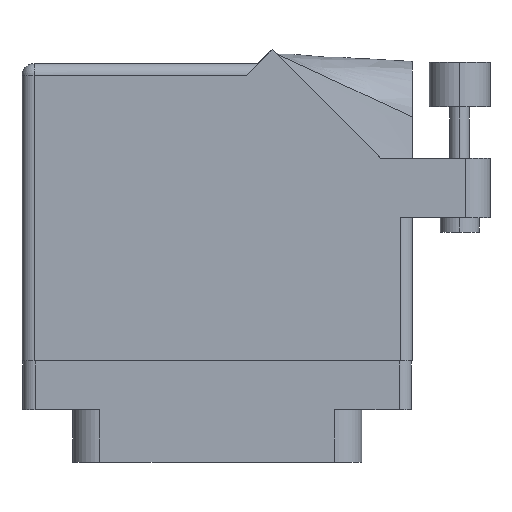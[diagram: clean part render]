
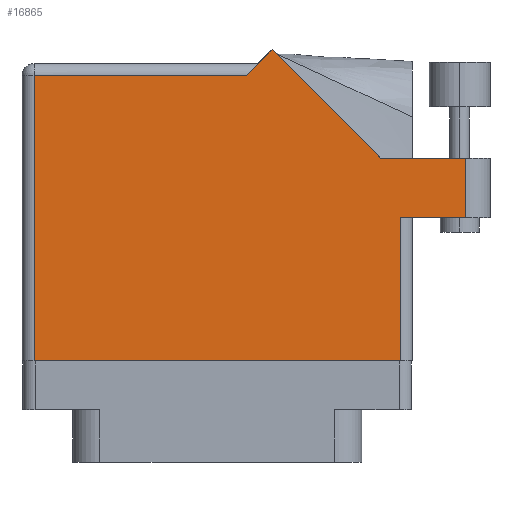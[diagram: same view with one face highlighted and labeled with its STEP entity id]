
A CAD part, front view. The second image highlights one B-rep face of the part: STEP entity #16865.
In plain terms, the highlighted face is planar.
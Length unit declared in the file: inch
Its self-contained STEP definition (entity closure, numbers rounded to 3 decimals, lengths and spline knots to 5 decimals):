
#17 = DIRECTION ( 'NONE',  ( -1., 0., 0. ) ) ;
#161 = VECTOR ( 'NONE', #27261, 39.37008 ) ;
#1463 = CARTESIAN_POINT ( 'NONE',  ( 1.405, 0.944, 0.455 ) ) ;
#2223 = VERTEX_POINT ( 'NONE', #5189 ) ;
#2932 = CARTESIAN_POINT ( 'NONE',  ( 0.83942, 0.944, 0.455 ) ) ;
#3528 = CARTESIAN_POINT ( 'NONE',  ( 1.28, 0.637, 0.455 ) ) ;
#3667 = VECTOR ( 'NONE', #25063, 39.37008 ) ;
#4051 = LINE ( 'NONE', #40041, #161 ) ;
#4214 = FACE_OUTER_BOUND ( 'NONE', #16245, .T. ) ;
#4226 = CARTESIAN_POINT ( 'NONE',  ( 0.943, 0.637, 0.455 ) ) ;
#4454 = DIRECTION ( 'NONE',  ( -1., 0., 0. ) ) ;
#4466 = CARTESIAN_POINT ( 'NONE',  ( 0.15, 1.368, 0.455 ) ) ;
#4490 = EDGE_CURVE ( 'NONE', #36131, #19155, #18329, .T. ) ;
#5189 = CARTESIAN_POINT ( 'NONE',  ( -0.943, 1.368, 0.455 ) ) ;
#6384 = VERTEX_POINT ( 'NONE', #32103 ) ;
#6926 = VERTEX_POINT ( 'NONE', #20071 ) ;
#7021 = VECTOR ( 'NONE', #33291, 39.37008 ) ;
#7250 = ORIENTED_EDGE ( 'NONE', *, *, #4490, .T. ) ;
#8870 = EDGE_CURVE ( 'NONE', #21446, #2223, #4051, .T. ) ;
#8940 = EDGE_CURVE ( 'NONE', #39528, #6384, #28328, .T. ) ;
#10396 = ORIENTED_EDGE ( 'NONE', *, *, #32902, .T. ) ;
#11553 = EDGE_CURVE ( 'NONE', #19155, #21446, #32974, .T. ) ;
#13306 = DIRECTION ( 'NONE',  ( -0.707, -0.707, 0. ) ) ;
#13759 = ORIENTED_EDGE ( 'NONE', *, *, #15859, .T. ) ;
#14920 = VERTEX_POINT ( 'NONE', #26353 ) ;
#15398 = ORIENTED_EDGE ( 'NONE', *, *, #8870, .T. ) ;
#15599 = PLANE ( 'NONE',  #40163 ) ;
#15859 = EDGE_CURVE ( 'NONE', #14920, #34988, #20311, .T. ) ;
#16245 = EDGE_LOOP ( 'NONE', ( #18199, #21356, #18265, #7250, #24539, #15398, #27740, #10396, #13759 ) ) ;
#16865 = ADVANCED_FACE ( 'NONE', ( #4214 ), #15599, .F. ) ;
#16963 = LINE ( 'NONE', #31550, #29628 ) ;
#17164 = DIRECTION ( 'NONE',  ( -0.707, 0.707, 0. ) ) ;
#17356 = EDGE_CURVE ( 'NONE', #34988, #39528, #27983, .T. ) ;
#18199 = ORIENTED_EDGE ( 'NONE', *, *, #17356, .T. ) ;
#18265 = ORIENTED_EDGE ( 'NONE', *, *, #26568, .T. ) ;
#18314 = LINE ( 'NONE', #1463, #38742 ) ;
#18329 = LINE ( 'NONE', #26810, #19810 ) ;
#19155 = VERTEX_POINT ( 'NONE', #21959 ) ;
#19273 = CARTESIAN_POINT ( 'NONE',  ( 0.943, 0.637, 0.455 ) ) ;
#19670 = DIRECTION ( 'NONE',  ( 0., 1., 0. ) ) ;
#19810 = VECTOR ( 'NONE', #17164, 39.37008 ) ;
#20071 = CARTESIAN_POINT ( 'NONE',  ( -0.943, -0.1, 0.455 ) ) ;
#20311 = LINE ( 'NONE', #19273, #31012 ) ;
#20610 = LINE ( 'NONE', #21045, #7021 ) ;
#21045 = CARTESIAN_POINT ( 'NONE',  ( -0.943, -0.1, 0.455 ) ) ;
#21356 = ORIENTED_EDGE ( 'NONE', *, *, #8940, .T. ) ;
#21446 = VERTEX_POINT ( 'NONE', #4466 ) ;
#21959 = CARTESIAN_POINT ( 'NONE',  ( 0.28271, 1.50071, 0.455 ) ) ;
#24539 = ORIENTED_EDGE ( 'NONE', *, *, #11553, .T. ) ;
#25014 = DIRECTION ( 'NONE',  ( 1., 0., 0. ) ) ;
#25063 = DIRECTION ( 'NONE',  ( 1., 0., 0. ) ) ;
#25674 = CARTESIAN_POINT ( 'NONE',  ( 0.212, 1.43, 0.455 ) ) ;
#26353 = CARTESIAN_POINT ( 'NONE',  ( 0.943, -0.1, 0.455 ) ) ;
#26568 = EDGE_CURVE ( 'NONE', #6384, #36131, #18314, .T. ) ;
#26810 = CARTESIAN_POINT ( 'NONE',  ( 0.83942, 0.944, 0.455 ) ) ;
#27261 = DIRECTION ( 'NONE',  ( -1., 0., 0. ) ) ;
#27740 = ORIENTED_EDGE ( 'NONE', *, *, #38437, .T. ) ;
#27983 = LINE ( 'NONE', #28462, #3667 ) ;
#28328 = LINE ( 'NONE', #37324, #29767 ) ;
#28462 = CARTESIAN_POINT ( 'NONE',  ( 1.005, 0.637, 0.455 ) ) ;
#29628 = VECTOR ( 'NONE', #25014, 39.37008 ) ;
#29767 = VECTOR ( 'NONE', #34321, 39.37008 ) ;
#31012 = VECTOR ( 'NONE', #19670, 39.37008 ) ;
#31372 = DIRECTION ( 'NONE',  ( 0., 0., -1. ) ) ;
#31548 = VECTOR ( 'NONE', #13306, 39.37008 ) ;
#31550 = CARTESIAN_POINT ( 'NONE',  ( -1.005, -0.1, 0.455 ) ) ;
#32103 = CARTESIAN_POINT ( 'NONE',  ( 1.28, 0.944, 0.455 ) ) ;
#32902 = EDGE_CURVE ( 'NONE', #6926, #14920, #16963, .T. ) ;
#32974 = LINE ( 'NONE', #25674, #31548 ) ;
#33291 = DIRECTION ( 'NONE',  ( 0., -1., 0. ) ) ;
#34321 = DIRECTION ( 'NONE',  ( 0., 1., 0. ) ) ;
#34988 = VERTEX_POINT ( 'NONE', #4226 ) ;
#36131 = VERTEX_POINT ( 'NONE', #2932 ) ;
#37324 = CARTESIAN_POINT ( 'NONE',  ( 1.28, 0.944, 0.455 ) ) ;
#38437 = EDGE_CURVE ( 'NONE', #2223, #6926, #20610, .T. ) ;
#38742 = VECTOR ( 'NONE', #4454, 39.37008 ) ;
#39528 = VERTEX_POINT ( 'NONE', #3528 ) ;
#40041 = CARTESIAN_POINT ( 'NONE',  ( -1.005, 1.368, 0.455 ) ) ;
#40163 = AXIS2_PLACEMENT_3D ( 'NONE', #40198, #31372, #17 ) ;
#40198 = CARTESIAN_POINT ( 'NONE',  ( -1.005, 1.43, 0.455 ) ) ;
